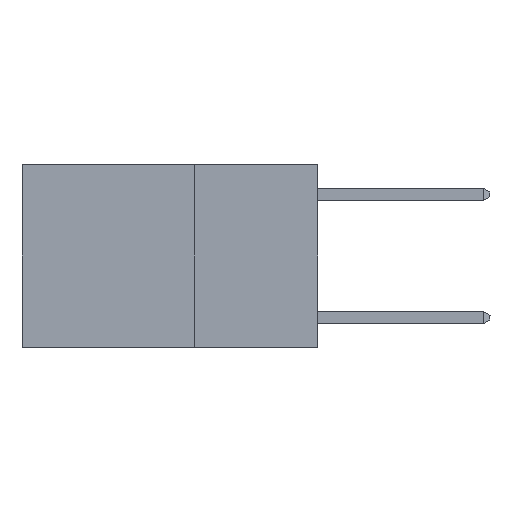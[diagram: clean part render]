
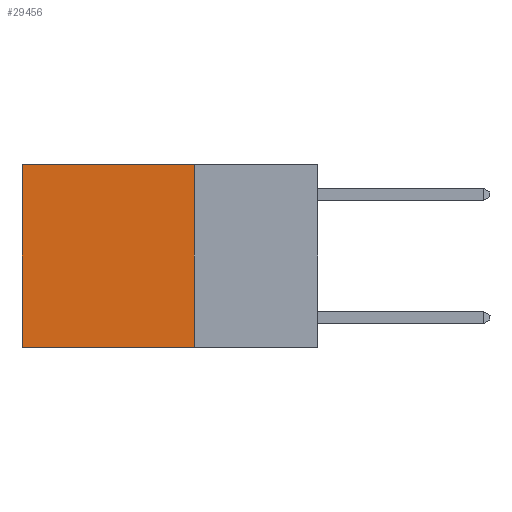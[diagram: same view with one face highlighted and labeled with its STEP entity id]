
A CAD part, left-side view. The second image highlights one B-rep face of the part: STEP entity #29456.
In plain terms, the highlighted planar face has unit normal (-1, 0, 0).
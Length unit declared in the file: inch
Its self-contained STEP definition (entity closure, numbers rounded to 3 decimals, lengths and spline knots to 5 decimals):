
#637 = FACE_OUTER_BOUND ( 'NONE', #3732, .T. ) ;
#878 = VECTOR ( 'NONE', #4139, 39.37008 ) ;
#1232 = CARTESIAN_POINT ( 'NONE',  ( 0.2625, 0.25, -0.37 ) ) ;
#1740 = DIRECTION ( 'NONE',  ( 0., 0., -1. ) ) ;
#1817 = CARTESIAN_POINT ( 'NONE',  ( 0.2625, 0.6, -0.37 ) ) ;
#3732 = EDGE_LOOP ( 'NONE', ( #14841, #6694, #12838, #25584 ) ) ;
#4139 = DIRECTION ( 'NONE',  ( 0., 0., -1. ) ) ;
#4753 = CARTESIAN_POINT ( 'NONE',  ( 0.2625, 0.25, 0. ) ) ;
#5882 = VERTEX_POINT ( 'NONE', #27860 ) ;
#6327 = LINE ( 'NONE', #8754, #878 ) ;
#6694 = ORIENTED_EDGE ( 'NONE', *, *, #6827, .F. ) ;
#6827 = EDGE_CURVE ( 'NONE', #17254, #14280, #20135, .T. ) ;
#7125 = AXIS2_PLACEMENT_3D ( 'NONE', #29037, #15611, #1740 ) ;
#8335 = LINE ( 'NONE', #10960, #20564 ) ;
#8605 = VECTOR ( 'NONE', #15152, 39.37008 ) ;
#8704 = LINE ( 'NONE', #21995, #26204 ) ;
#8754 = CARTESIAN_POINT ( 'NONE',  ( 0.2625, 0.6, 0. ) ) ;
#10610 = DIRECTION ( 'NONE',  ( 0., 1., 0. ) ) ;
#10960 = CARTESIAN_POINT ( 'NONE',  ( 0.2625, 0.25, 0. ) ) ;
#10976 = PLANE ( 'NONE',  #7125 ) ;
#12838 = ORIENTED_EDGE ( 'NONE', *, *, #26950, .F. ) ;
#14280 = VERTEX_POINT ( 'NONE', #1817 ) ;
#14841 = ORIENTED_EDGE ( 'NONE', *, *, #20542, .T. ) ;
#15152 = DIRECTION ( 'NONE',  ( 0., 1., 0. ) ) ;
#15611 = DIRECTION ( 'NONE',  ( 1., 0., 0. ) ) ;
#17254 = VERTEX_POINT ( 'NONE', #25620 ) ;
#20135 = LINE ( 'NONE', #1232, #8605 ) ;
#20542 = EDGE_CURVE ( 'NONE', #5882, #14280, #6327, .T. ) ;
#20564 = VECTOR ( 'NONE', #29027, 39.37008 ) ;
#21995 = CARTESIAN_POINT ( 'NONE',  ( 0.2625, 0.25, 0. ) ) ;
#22167 = VERTEX_POINT ( 'NONE', #4753 ) ;
#22511 = EDGE_CURVE ( 'NONE', #22167, #5882, #8704, .T. ) ;
#25584 = ORIENTED_EDGE ( 'NONE', *, *, #22511, .T. ) ;
#25620 = CARTESIAN_POINT ( 'NONE',  ( 0.2625, 0.25, -0.37 ) ) ;
#26204 = VECTOR ( 'NONE', #10610, 39.37008 ) ;
#26950 = EDGE_CURVE ( 'NONE', #22167, #17254, #8335, .T. ) ;
#27860 = CARTESIAN_POINT ( 'NONE',  ( 0.2625, 0.6, 0. ) ) ;
#29027 = DIRECTION ( 'NONE',  ( 0., 0., -1. ) ) ;
#29037 = CARTESIAN_POINT ( 'NONE',  ( 0.2625, 0.25, 0. ) ) ;
#29456 = ADVANCED_FACE ( 'NONE', ( #637 ), #10976, .F. ) ;
